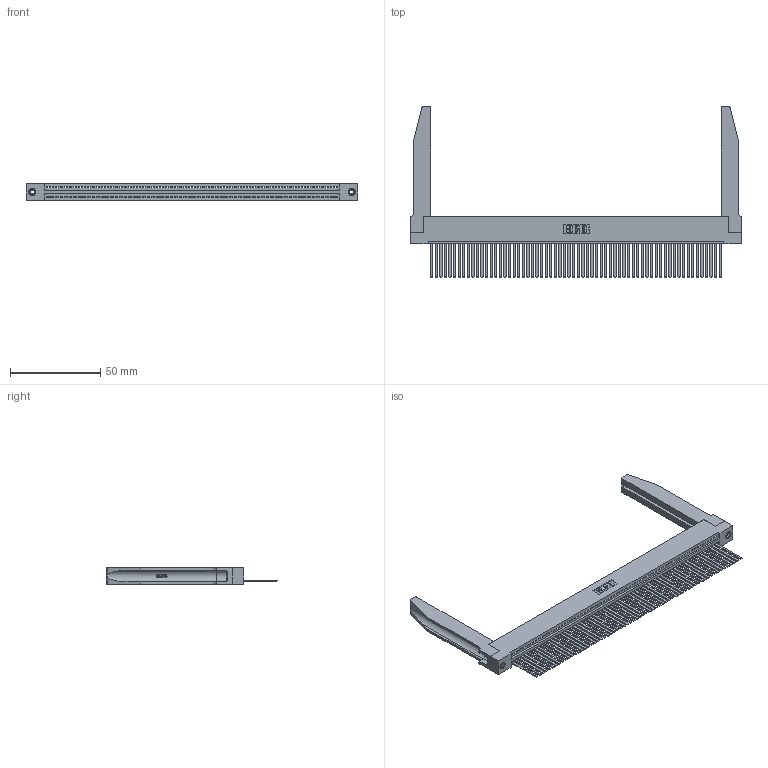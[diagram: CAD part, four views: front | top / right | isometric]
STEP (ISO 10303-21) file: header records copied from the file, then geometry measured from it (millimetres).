
FILE_DESCRIPTION (( 'STEP AP203' ), '1' );
FILE_NAME ('395-064-544-178.STEP', '2019-10-25T03:17:32', ( '' ), ( '' ), 'SwSTEP 2.0', 'SolidWorks 2016', '' );
FILE_SCHEMA (( 'CONFIG_CONTROL_DESIGN' ));
Length unit declared in the file: inch
Products named in the file (5): 345-292-001_345-293-144; 345-220-078_345-220-078; 345 Part_Flush Mounting Lugs - 0.156 Dia-TH; 395-064-544-178; 345-250-001_345-250-001-102
Assembly tree (69 placements, depth 2):
  395-064-544-178
    345 Part_Flush Mounting Lugs - 0.156 Dia-TH
    345-292-001_345-293-144  x64
    345-250-001_345-250-001-102  x2
    345-220-078_345-220-078  x2
Bounding box: 183.79 x 94.92 x 9.4 mm (x, y, z)
Volume: 26148.9 mm3; surface area: 33793 mm2
Topology: 69 solids, 69 shells, 3688 faces, 11061 edges, 7278 vertices
Faces by surface type: plane 2526, cylinder 1110, bspline 36, cone 12, torus 4
Entity records: 49762 total; most frequent: CARTESIAN_POINT 9515, ORIENTED_EDGE 8410, DIRECTION 7283, EDGE_CURVE 4205, LINE 3727, VECTOR 3727, VERTEX_POINT 2796, AXIS2_PLACEMENT_3D 1778
